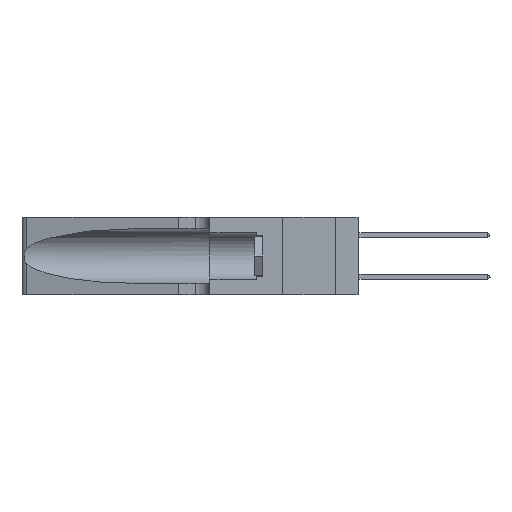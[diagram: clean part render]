
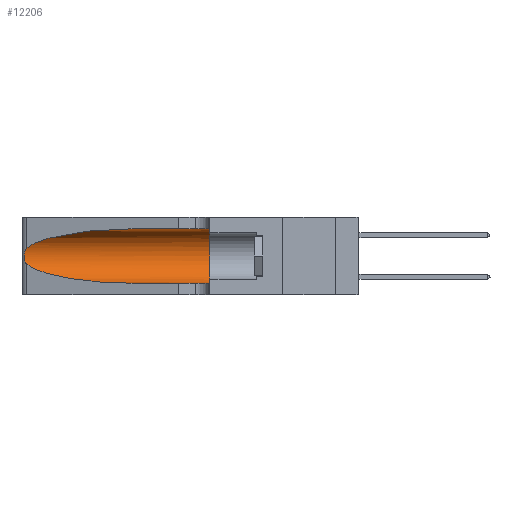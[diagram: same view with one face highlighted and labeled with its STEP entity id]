
A CAD part, left-side view. The second image highlights one B-rep face of the part: STEP entity #12206.
In plain terms, the highlighted cylindrical face has radius 3.308 mm (diameter 6.617 mm), a partial arc.
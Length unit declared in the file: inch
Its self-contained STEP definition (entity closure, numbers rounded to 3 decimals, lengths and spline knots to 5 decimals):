
#16 = EDGE_CURVE ( 'NONE', #20876, #4429, #14907, .T. ) ;
#951 = CARTESIAN_POINT ( 'NONE',  ( 0.26018, 1.23835, 0.19895 ) ) ;
#993 = CARTESIAN_POINT ( 'NONE',  ( 0.1305, 0.35, 0.05475 ) ) ;
#1065 = CARTESIAN_POINT ( 'NONE',  ( 0.25639, 1.23184, 0.21858 ) ) ;
#1406 = LINE ( 'NONE', #7850, #21363 ) ;
#1459 = LINE ( 'NONE', #6617, #6901 ) ;
#2414 = AXIS2_PLACEMENT_3D ( 'NONE', #16436, #4046, #25372 ) ;
#3249 = DIRECTION ( 'NONE',  ( 0., -1., 0. ) ) ;
#3310 = CARTESIAN_POINT ( 'NONE',  ( 0.25787, 1.23484, 0.2124 ) ) ;
#4046 = DIRECTION ( 'NONE',  ( 0., 1., 0. ) ) ;
#4346 = CYLINDRICAL_SURFACE ( 'NONE', #25889, 0.13025 ) ;
#4429 = VERTEX_POINT ( 'NONE', #10941 ) ;
#4510 = EDGE_CURVE ( 'NONE', #20876, #17530, #1459, .T. ) ;
#5166 = CARTESIAN_POINT ( 'NONE',  ( 0.25487, 1.22718, 0.14631 ) ) ;
#5622 = CARTESIAN_POINT ( 'NONE',  ( 0.26075, 1.23896, 0.178 ) ) ;
#6617 = CARTESIAN_POINT ( 'NONE',  ( 0.1305, 1.61858, 0.31525 ) ) ;
#6901 = VECTOR ( 'NONE', #11716, 39.37008 ) ;
#7119 = CARTESIAN_POINT ( 'NONE',  ( 0.18966, 0.96281, 0.05475 ) ) ;
#7146 = EDGE_CURVE ( 'NONE', #15613, #15651, #9463, .T. ) ;
#7850 = CARTESIAN_POINT ( 'NONE',  ( 0.1305, 1.61858, 0.05475 ) ) ;
#8410 = CARTESIAN_POINT ( 'NONE',  ( 0.25789, 1.23486, 0.15765 ) ) ;
#8756 = CARTESIAN_POINT ( 'NONE',  ( 0.2373, 1.15595, 0.28018 ) ) ;
#8850 = ORIENTED_EDGE ( 'NONE', *, *, #4510, .F. ) ;
#9463 =( BOUNDED_CURVE ( )  B_SPLINE_CURVE ( 3, ( #25486, #28986, #7119, #23678 ),
 .UNSPECIFIED., .F., .F. ) 
 B_SPLINE_CURVE_WITH_KNOTS ( ( 4, 4 ),
 ( 3.44316, 4.71239 ),
 .UNSPECIFIED. ) 
 CURVE ( )  GEOMETRIC_REPRESENTATION_ITEM ( )  RATIONAL_B_SPLINE_CURVE ( ( 1., 0.87, 0.87, 1. ) ) 
 REPRESENTATION_ITEM ( '' )  );
#9744 = ORIENTED_EDGE ( 'NONE', *, *, #15334, .T. ) ;
#10941 = CARTESIAN_POINT ( 'NONE',  ( 0.25487, 1.22718, 0.22369 ) ) ;
#11716 = DIRECTION ( 'NONE',  ( 0., -1., 0. ) ) ;
#12206 = ADVANCED_FACE ( 'NONE', ( #27406 ), #4346, .F. ) ;
#12518 = CARTESIAN_POINT ( 'NONE',  ( 0.1305, 1.61858, 0.185 ) ) ;
#13490 = CARTESIAN_POINT ( 'NONE',  ( 0.1305, 0.35, 0.31525 ) ) ;
#13766 = ORIENTED_EDGE ( 'NONE', *, *, #7146, .T. ) ;
#14472 = CIRCLE ( 'NONE', #2414, 0.13025 ) ;
#14907 =( BOUNDED_CURVE ( )  B_SPLINE_CURVE ( 3, ( #29468, #27433, #8756, #15892 ),
 .UNSPECIFIED., .F., .T. ) 
 B_SPLINE_CURVE_WITH_KNOTS ( ( 4, 4 ),
 ( 1.5708, 2.84003 ),
 .UNSPECIFIED. ) 
 CURVE ( )  GEOMETRIC_REPRESENTATION_ITEM ( )  RATIONAL_B_SPLINE_CURVE ( ( 1., 0.87, 0.87, 1. ) ) 
 REPRESENTATION_ITEM ( '' )  );
#15334 = EDGE_CURVE ( 'NONE', #4429, #15613, #20301, .T. ) ;
#15613 = VERTEX_POINT ( 'NONE', #5166 ) ;
#15651 = VERTEX_POINT ( 'NONE', #16785 ) ;
#15892 = CARTESIAN_POINT ( 'NONE',  ( 0.25487, 1.22718, 0.22369 ) ) ;
#16044 = EDGE_CURVE ( 'NONE', #17530, #22059, #14472, .T. ) ;
#16436 = CARTESIAN_POINT ( 'NONE',  ( 0.1305, 0.35, 0.185 ) ) ;
#16722 = EDGE_LOOP ( 'NONE', ( #29393, #9744, #13766, #19034, #26887, #8850 ) ) ;
#16785 = CARTESIAN_POINT ( 'NONE',  ( 0.1305, 0.72297, 0.05475 ) ) ;
#17530 = VERTEX_POINT ( 'NONE', #13490 ) ;
#18683 = EDGE_CURVE ( 'NONE', #15651, #22059, #1406, .T. ) ;
#19034 = ORIENTED_EDGE ( 'NONE', *, *, #18683, .T. ) ;
#19508 = CARTESIAN_POINT ( 'NONE',  ( 0.25639, 1.23186, 0.15144 ) ) ;
#19517 = DIRECTION ( 'NONE',  ( 0., 0., -1. ) ) ;
#19581 = CARTESIAN_POINT ( 'NONE',  ( 0.26075, 1.23896, 0.19203 ) ) ;
#20301 = B_SPLINE_CURVE_WITH_KNOTS ( 'NONE', 3,
 ( #21792, #26344, #1065, #3310, #24127, #951, #19581, #5622, #21902, #29217, #8410, #19508, #28821, #21941 ),
 .UNSPECIFIED., .F., .F.,
 ( 4, 2, 2, 2, 2, 2, 4 ),
 ( 0., 0.00027, 0.00053, 0.00107, 0.0016, 0.00187, 0.00214 ),
 .UNSPECIFIED. ) ;
#20876 = VERTEX_POINT ( 'NONE', #28894 ) ;
#21363 = VECTOR ( 'NONE', #28656, 39.37008 ) ;
#21792 = CARTESIAN_POINT ( 'NONE',  ( 0.25487, 1.22718, 0.22369 ) ) ;
#21902 = CARTESIAN_POINT ( 'NONE',  ( 0.26017, 1.23833, 0.17102 ) ) ;
#21941 = CARTESIAN_POINT ( 'NONE',  ( 0.25487, 1.22718, 0.14631 ) ) ;
#22059 = VERTEX_POINT ( 'NONE', #993 ) ;
#23678 = CARTESIAN_POINT ( 'NONE',  ( 0.1305, 0.72297, 0.05475 ) ) ;
#24127 = CARTESIAN_POINT ( 'NONE',  ( 0.25854, 1.2359, 0.20912 ) ) ;
#25372 = DIRECTION ( 'NONE',  ( 0., 0., 1. ) ) ;
#25486 = CARTESIAN_POINT ( 'NONE',  ( 0.25487, 1.22718, 0.14631 ) ) ;
#25889 = AXIS2_PLACEMENT_3D ( 'NONE', #12518, #3249, #19517 ) ;
#26344 = CARTESIAN_POINT ( 'NONE',  ( 0.25555, 1.22994, 0.2215 ) ) ;
#26887 = ORIENTED_EDGE ( 'NONE', *, *, #16044, .F. ) ;
#27406 = FACE_OUTER_BOUND ( 'NONE', #16722, .T. ) ;
#27433 = CARTESIAN_POINT ( 'NONE',  ( 0.18966, 0.96281, 0.31525 ) ) ;
#28656 = DIRECTION ( 'NONE',  ( 0., -1., 0. ) ) ;
#28821 = CARTESIAN_POINT ( 'NONE',  ( 0.25555, 1.22993, 0.14849 ) ) ;
#28894 = CARTESIAN_POINT ( 'NONE',  ( 0.1305, 0.72297, 0.31525 ) ) ;
#28986 = CARTESIAN_POINT ( 'NONE',  ( 0.2373, 1.15595, 0.08982 ) ) ;
#29217 = CARTESIAN_POINT ( 'NONE',  ( 0.25856, 1.23593, 0.16098 ) ) ;
#29393 = ORIENTED_EDGE ( 'NONE', *, *, #16, .T. ) ;
#29468 = CARTESIAN_POINT ( 'NONE',  ( 0.1305, 0.72297, 0.31525 ) ) ;
